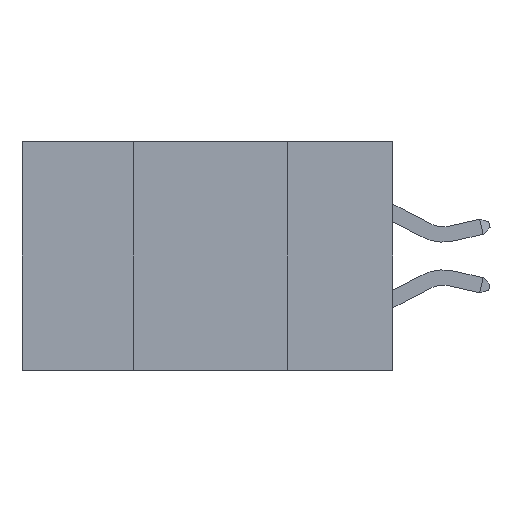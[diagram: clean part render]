
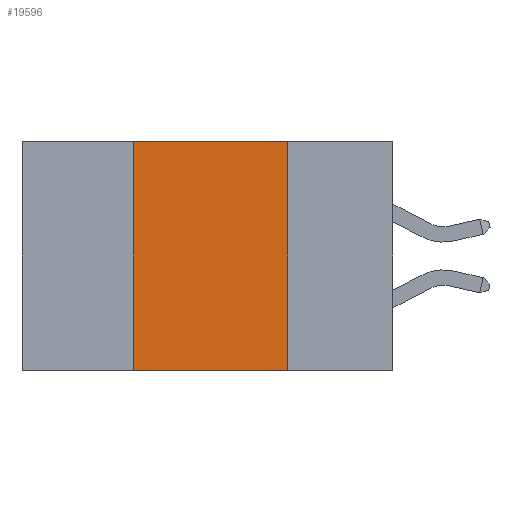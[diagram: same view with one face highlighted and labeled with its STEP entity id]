
A CAD part, left-side view. The second image highlights one B-rep face of the part: STEP entity #19596.
In plain terms, the highlighted planar face has unit normal (-1, 0, 0).
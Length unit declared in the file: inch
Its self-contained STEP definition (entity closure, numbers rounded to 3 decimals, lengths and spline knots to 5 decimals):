
#42 = EDGE_LOOP ( 'NONE', ( #19623, #4442, #25740, #10427 ) ) ;
#518 = DIRECTION ( 'NONE',  ( 0., 0., 1. ) ) ;
#648 = VERTEX_POINT ( 'NONE', #13377 ) ;
#3097 = DIRECTION ( 'NONE',  ( 1., 0., 0. ) ) ;
#3127 = CARTESIAN_POINT ( 'NONE',  ( 0., 0.17, 0. ) ) ;
#3191 = LINE ( 'NONE', #19681, #18188 ) ;
#3318 = DIRECTION ( 'NONE',  ( 0., -1., 0. ) ) ;
#4442 = ORIENTED_EDGE ( 'NONE', *, *, #29185, .F. ) ;
#5351 = DIRECTION ( 'NONE',  ( 0., -1., 0. ) ) ;
#5641 = DIRECTION ( 'NONE',  ( 0., 0., -1. ) ) ;
#5839 = EDGE_CURVE ( 'NONE', #17841, #10055, #3191, .T. ) ;
#7108 = VECTOR ( 'NONE', #518, 39.37008 ) ;
#9352 = LINE ( 'NONE', #25847, #7108 ) ;
#10055 = VERTEX_POINT ( 'NONE', #26641 ) ;
#10427 = ORIENTED_EDGE ( 'NONE', *, *, #20660, .T. ) ;
#13377 = CARTESIAN_POINT ( 'NONE',  ( 0., 0.42, -0.37 ) ) ;
#14170 = CARTESIAN_POINT ( 'NONE',  ( 0., 0.6, -0.37 ) ) ;
#14684 = FACE_OUTER_BOUND ( 'NONE', #42, .T. ) ;
#17071 = CARTESIAN_POINT ( 'NONE',  ( 0., 0.6, 0. ) ) ;
#17841 = VERTEX_POINT ( 'NONE', #3127 ) ;
#18188 = VECTOR ( 'NONE', #5641, 39.37008 ) ;
#18789 = LINE ( 'NONE', #14170, #19221 ) ;
#19148 = PLANE ( 'NONE',  #25551 ) ;
#19221 = VECTOR ( 'NONE', #5351, 39.37008 ) ;
#19387 = VECTOR ( 'NONE', #3318, 39.37008 ) ;
#19596 = ADVANCED_FACE ( 'NONE', ( #14684 ), #19148, .F. ) ;
#19623 = ORIENTED_EDGE ( 'NONE', *, *, #5839, .F. ) ;
#19681 = CARTESIAN_POINT ( 'NONE',  ( 0., 0.17, 0. ) ) ;
#20660 = EDGE_CURVE ( 'NONE', #648, #10055, #18789, .T. ) ;
#21597 = CARTESIAN_POINT ( 'NONE',  ( 0., 0.6, 0. ) ) ;
#24431 = LINE ( 'NONE', #17071, #19387 ) ;
#25267 = VERTEX_POINT ( 'NONE', #27081 ) ;
#25551 = AXIS2_PLACEMENT_3D ( 'NONE', #21597, #3097, #28551 ) ;
#25740 = ORIENTED_EDGE ( 'NONE', *, *, #30334, .F. ) ;
#25847 = CARTESIAN_POINT ( 'NONE',  ( 0., 0.42, 0. ) ) ;
#26641 = CARTESIAN_POINT ( 'NONE',  ( 0., 0.17, -0.37 ) ) ;
#27081 = CARTESIAN_POINT ( 'NONE',  ( 0., 0.42, 0. ) ) ;
#28551 = DIRECTION ( 'NONE',  ( 0., 0., -1. ) ) ;
#29185 = EDGE_CURVE ( 'NONE', #25267, #17841, #24431, .T. ) ;
#30334 = EDGE_CURVE ( 'NONE', #648, #25267, #9352, .T. ) ;
